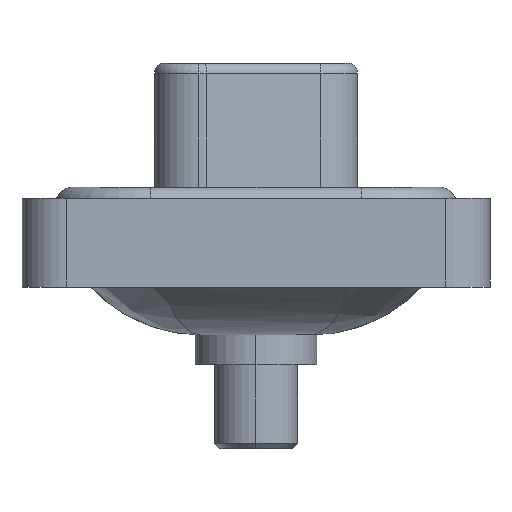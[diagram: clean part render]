
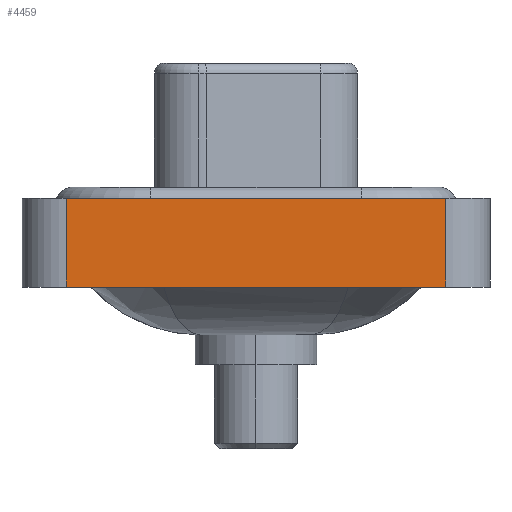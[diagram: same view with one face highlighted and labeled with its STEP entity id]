
A CAD part, left-side view. The second image highlights one B-rep face of the part: STEP entity #4459.
In plain terms, the highlighted planar face has unit normal (-1, 0, 0).
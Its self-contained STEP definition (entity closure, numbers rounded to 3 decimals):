
#585 = LINE ( 'NONE', #1832, #9370 ) ;
#856 = CARTESIAN_POINT ( 'NONE',  ( -7.25, -8.55, -3.6 ) ) ;
#1076 = LINE ( 'NONE', #15992, #16122 ) ;
#1138 = EDGE_CURVE ( 'NONE', #3725, #5169, #1076, .T. ) ;
#1618 = DIRECTION ( 'NONE',  ( -1., 0., 0. ) ) ;
#1832 = CARTESIAN_POINT ( 'NONE',  ( -7.25, -8.55, 0.4 ) ) ;
#1993 = ORIENTED_EDGE ( 'NONE', *, *, #14337, .T. ) ;
#2448 = AXIS2_PLACEMENT_3D ( 'NONE', #15034, #1618, #4228 ) ;
#2795 = LINE ( 'NONE', #11274, #15064 ) ;
#3195 = EDGE_CURVE ( 'NONE', #15012, #11471, #2795, .T. ) ;
#3725 = VERTEX_POINT ( 'NONE', #11349 ) ;
#4228 = DIRECTION ( 'NONE',  ( 0., 0., 1. ) ) ;
#4389 = FACE_OUTER_BOUND ( 'NONE', #6754, .T. ) ;
#4459 = ADVANCED_FACE ( 'NONE', ( #4389 ), #9594, .T. ) ;
#4496 = ORIENTED_EDGE ( 'NONE', *, *, #12439, .F. ) ;
#5169 = VERTEX_POINT ( 'NONE', #17507 ) ;
#5291 = DIRECTION ( 'NONE',  ( 0., 0., 1. ) ) ;
#6754 = EDGE_LOOP ( 'NONE', ( #12766, #4496, #14414, #1993 ) ) ;
#7129 = DIRECTION ( 'NONE',  ( 0., -1., 0. ) ) ;
#8331 = DIRECTION ( 'NONE',  ( 0., 0., 1. ) ) ;
#9370 = VECTOR ( 'NONE', #7129, 1000. ) ;
#9594 = PLANE ( 'NONE',  #2448 ) ;
#10340 = LINE ( 'NONE', #856, #13118 ) ;
#10669 = CARTESIAN_POINT ( 'NONE',  ( -7.25, -8.55, -3.6 ) ) ;
#11274 = CARTESIAN_POINT ( 'NONE',  ( -7.25, -8.55, -3.6 ) ) ;
#11349 = CARTESIAN_POINT ( 'NONE',  ( -7.25, 8.55, -3.6 ) ) ;
#11471 = VERTEX_POINT ( 'NONE', #16826 ) ;
#12439 = EDGE_CURVE ( 'NONE', #5169, #11471, #585, .T. ) ;
#12766 = ORIENTED_EDGE ( 'NONE', *, *, #3195, .T. ) ;
#13118 = VECTOR ( 'NONE', #17042, 1000. ) ;
#14337 = EDGE_CURVE ( 'NONE', #3725, #15012, #10340, .T. ) ;
#14414 = ORIENTED_EDGE ( 'NONE', *, *, #1138, .F. ) ;
#15012 = VERTEX_POINT ( 'NONE', #10669 ) ;
#15034 = CARTESIAN_POINT ( 'NONE',  ( -7.25, -8.55, -3.6 ) ) ;
#15064 = VECTOR ( 'NONE', #8331, 1000. ) ;
#15992 = CARTESIAN_POINT ( 'NONE',  ( -7.25, 8.55, -3.6 ) ) ;
#16122 = VECTOR ( 'NONE', #5291, 1000. ) ;
#16826 = CARTESIAN_POINT ( 'NONE',  ( -7.25, -8.55, 0.4 ) ) ;
#17042 = DIRECTION ( 'NONE',  ( 0., -1., 0. ) ) ;
#17507 = CARTESIAN_POINT ( 'NONE',  ( -7.25, 8.55, 0.4 ) ) ;
